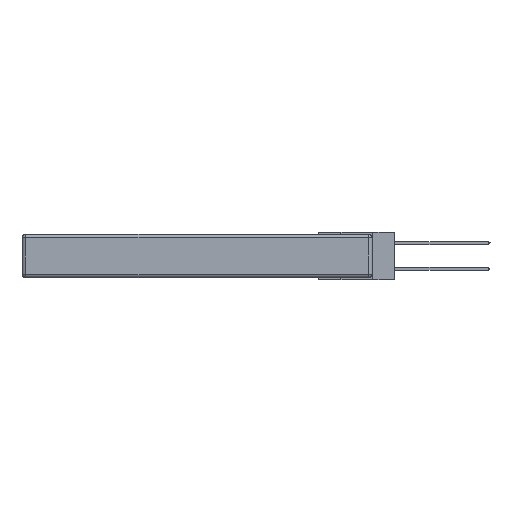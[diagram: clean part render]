
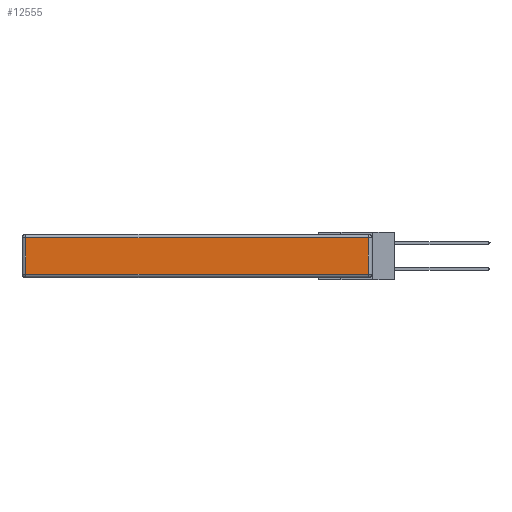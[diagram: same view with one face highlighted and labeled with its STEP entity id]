
A CAD part, left-side view. The second image highlights one B-rep face of the part: STEP entity #12555.
In plain terms, the highlighted planar face has unit normal (-1, 0, 0).
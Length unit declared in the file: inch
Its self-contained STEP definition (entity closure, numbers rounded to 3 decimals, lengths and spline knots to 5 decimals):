
#656 = DIRECTION ( 'NONE',  ( 0., -1., 0. ) ) ;
#782 = VECTOR ( 'NONE', #23947, 39.37008 ) ;
#822 = CARTESIAN_POINT ( 'NONE',  ( 0., 0.03, -0.343 ) ) ;
#1321 = CARTESIAN_POINT ( 'NONE',  ( 0., 2.72, -0.313 ) ) ;
#3126 = CARTESIAN_POINT ( 'NONE',  ( 0., 0., -0.343 ) ) ;
#3428 = LINE ( 'NONE', #16796, #6287 ) ;
#4407 = DIRECTION ( 'NONE',  ( 0., 1., 0. ) ) ;
#4459 = EDGE_CURVE ( 'NONE', #20717, #25707, #25162, .T. ) ;
#4960 = VECTOR ( 'NONE', #4407, 39.37008 ) ;
#6254 = CARTESIAN_POINT ( 'NONE',  ( 0., 0.03, -0.313 ) ) ;
#6262 = AXIS2_PLACEMENT_3D ( 'NONE', #3126, #7726, #14158 ) ;
#6287 = VECTOR ( 'NONE', #656, 39.37008 ) ;
#7628 = DIRECTION ( 'NONE',  ( 0., 0., 1. ) ) ;
#7632 = ORIENTED_EDGE ( 'NONE', *, *, #26094, .T. ) ;
#7726 = DIRECTION ( 'NONE',  ( -1., 0., 0. ) ) ;
#8281 = EDGE_CURVE ( 'NONE', #22255, #20717, #11343, .T. ) ;
#9991 = VERTEX_POINT ( 'NONE', #6254 ) ;
#10485 = VECTOR ( 'NONE', #7628, 39.37008 ) ;
#11343 = LINE ( 'NONE', #27363, #4960 ) ;
#12555 = ADVANCED_FACE ( 'NONE', ( #27314 ), #27190, .T. ) ;
#13092 = ORIENTED_EDGE ( 'NONE', *, *, #18303, .T. ) ;
#14158 = DIRECTION ( 'NONE',  ( 0., 0., 1. ) ) ;
#14634 = CARTESIAN_POINT ( 'NONE',  ( 0., 2.72, -0.343 ) ) ;
#16796 = CARTESIAN_POINT ( 'NONE',  ( 0., 0., -0.313 ) ) ;
#18061 = ORIENTED_EDGE ( 'NONE', *, *, #4459, .T. ) ;
#18303 = EDGE_CURVE ( 'NONE', #9991, #22255, #23804, .T. ) ;
#20717 = VERTEX_POINT ( 'NONE', #23381 ) ;
#22255 = VERTEX_POINT ( 'NONE', #29227 ) ;
#22844 = EDGE_LOOP ( 'NONE', ( #7632, #13092, #27528, #18061 ) ) ;
#23381 = CARTESIAN_POINT ( 'NONE',  ( 0., 2.72, -0.03 ) ) ;
#23804 = LINE ( 'NONE', #822, #10485 ) ;
#23947 = DIRECTION ( 'NONE',  ( 0., 0., -1. ) ) ;
#25162 = LINE ( 'NONE', #14634, #782 ) ;
#25707 = VERTEX_POINT ( 'NONE', #1321 ) ;
#26094 = EDGE_CURVE ( 'NONE', #25707, #9991, #3428, .T. ) ;
#27190 = PLANE ( 'NONE',  #6262 ) ;
#27314 = FACE_OUTER_BOUND ( 'NONE', #22844, .T. ) ;
#27363 = CARTESIAN_POINT ( 'NONE',  ( 0., 2.75, -0.03 ) ) ;
#27528 = ORIENTED_EDGE ( 'NONE', *, *, #8281, .T. ) ;
#29227 = CARTESIAN_POINT ( 'NONE',  ( 0., 0.03, -0.03 ) ) ;
